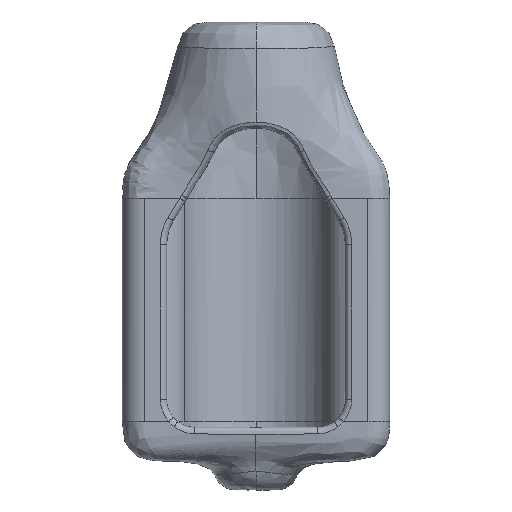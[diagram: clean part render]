
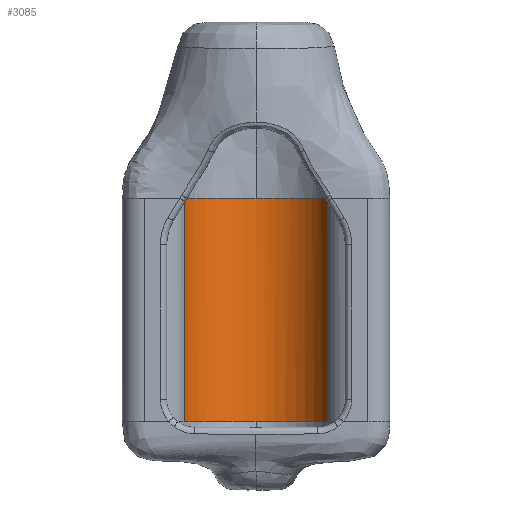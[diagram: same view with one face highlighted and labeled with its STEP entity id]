
A CAD part, front view. The second image highlights one B-rep face of the part: STEP entity #3085.
In plain terms, the highlighted cylindrical face has radius 5.334 mm (diameter 10.668 mm), a partial arc.
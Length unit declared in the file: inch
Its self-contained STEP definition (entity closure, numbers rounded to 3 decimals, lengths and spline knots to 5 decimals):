
#1007 = CARTESIAN_POINT ( 'NONE',  ( -0.13242, 0.16425, 0.3 ) ) ;
#1237 = CARTESIAN_POINT ( 'NONE',  ( -0.09839, 0.18664, 0.3 ) ) ;
#2120 = ORIENTED_EDGE ( 'NONE', *, *, #5788, .F. ) ;
#2580 = B_SPLINE_CURVE_WITH_KNOTS ( 'NONE', 3,
 ( #12126, #18629, #8421, #4940, #1237, #1007, #15390, #19093, #15161, #11673 ),
 .UNSPECIFIED., .F., .F.,
 ( 4, 2, 2, 2, 4 ),
 ( 0., 0.25, 0.5, 0.75, 1. ),
 .UNSPECIFIED. ) ;
#3085 = ADVANCED_FACE ( 'NONE', ( #8652 ), #4949, .F. ) ;
#3102 = CARTESIAN_POINT ( 'NONE',  ( -0.19284, 0.08315, 0. ) ) ;
#3158 = CARTESIAN_POINT ( 'NONE',  ( -0.17781, 0.11334, -0.3 ) ) ;
#3614 = CARTESIAN_POINT ( 'NONE',  ( -0.10339, 0.18471, -0.3 ) ) ;
#4940 = CARTESIAN_POINT ( 'NONE',  ( -0.07974, 0.19533, 0.3 ) ) ;
#4949 = CYLINDRICAL_SURFACE ( 'NONE', #31239, 0.21 ) ;
#5514 = CARTESIAN_POINT ( 'NONE',  ( 0.14779, 0.15057, 0.3 ) ) ;
#5788 = EDGE_CURVE ( 'NONE', #8398, #17415, #29320, .T. ) ;
#6465 = CARTESIAN_POINT ( 'NONE',  ( 0.19284, 0.08315, 0.3 ) ) ;
#8117 = VERTEX_POINT ( 'NONE', #12225 ) ;
#8315 = CARTESIAN_POINT ( 'NONE',  ( 0., 0.21, 0.3 ) ) ;
#8361 = EDGE_CURVE ( 'NONE', #17415, #32532, #33169, .T. ) ;
#8390 = ORIENTED_EDGE ( 'NONE', *, *, #43755, .T. ) ;
#8398 = VERTEX_POINT ( 'NONE', #17536 ) ;
#8421 = CARTESIAN_POINT ( 'NONE',  ( -0.04073, 0.20702, 0.3 ) ) ;
#8652 = FACE_OUTER_BOUND ( 'NONE', #40180, .T. ) ;
#8676 = B_SPLINE_CURVE_WITH_KNOTS ( 'NONE', 3,
 ( #37296, #40773, #43806, #5514, #16187, #44489, #39868, #43579, #36384, #8315 ),
 .UNSPECIFIED., .F., .F.,
 ( 4, 2, 2, 2, 4 ),
 ( 0., 0.25, 0.5, 0.75, 1. ),
 .UNSPECIFIED. ) ;
#8844 = ORIENTED_EDGE ( 'NONE', *, *, #27323, .T. ) ;
#9076 = CARTESIAN_POINT ( 'NONE',  ( 0.18831, 0.09364, -0.3 ) ) ;
#11673 = CARTESIAN_POINT ( 'NONE',  ( -0.19284, 0.08315, 0.3 ) ) ;
#12126 = CARTESIAN_POINT ( 'NONE',  ( 0., 0.21, 0.3 ) ) ;
#12184 = CARTESIAN_POINT ( 'NONE',  ( 0.19284, 0.08315, 0. ) ) ;
#12225 = CARTESIAN_POINT ( 'NONE',  ( -0.19284, 0.08315, 0.3 ) ) ;
#12360 = DIRECTION ( 'NONE',  ( 1., 0., 0. ) ) ;
#13601 = CARTESIAN_POINT ( 'NONE',  ( -0.18831, 0.09364, -0.3 ) ) ;
#14013 = LINE ( 'NONE', #3102, #37925 ) ;
#15161 = CARTESIAN_POINT ( 'NONE',  ( -0.18477, 0.10185, 0.3 ) ) ;
#15390 = CARTESIAN_POINT ( 'NONE',  ( -0.14779, 0.15057, 0.3 ) ) ;
#16187 = CARTESIAN_POINT ( 'NONE',  ( 0.13242, 0.16425, 0.3 ) ) ;
#16733 = CARTESIAN_POINT ( 'NONE',  ( 0.17781, 0.11334, -0.3 ) ) ;
#16959 = CARTESIAN_POINT ( 'NONE',  ( 0.01932, 0.21, -0.3 ) ) ;
#17415 = VERTEX_POINT ( 'NONE', #38245 ) ;
#17536 = CARTESIAN_POINT ( 'NONE',  ( 0.19284, 0.08315, -0.3 ) ) ;
#17591 = VERTEX_POINT ( 'NONE', #6465 ) ;
#18629 = CARTESIAN_POINT ( 'NONE',  ( -0.02036, 0.21, 0.3 ) ) ;
#18925 = CARTESIAN_POINT ( 'NONE',  ( -0.19284, 0.08315, -0.3 ) ) ;
#19093 = CARTESIAN_POINT ( 'NONE',  ( -0.17397, 0.11937, 0.3 ) ) ;
#19153 = LINE ( 'NONE', #12184, #31270 ) ;
#20446 = CARTESIAN_POINT ( 'NONE',  ( 0.05795, 0.20467, -0.3 ) ) ;
#20845 = ORIENTED_EDGE ( 'NONE', *, *, #8361, .F. ) ;
#21021 = CARTESIAN_POINT ( 'NONE',  ( -0.15842, 0.13904, -0.3 ) ) ;
#21658 = DIRECTION ( 'NONE',  ( 0., 0., 1. ) ) ;
#23000 = CARTESIAN_POINT ( 'NONE',  ( 0., 0.21, -0.3 ) ) ;
#24727 = CARTESIAN_POINT ( 'NONE',  ( -0.13617, 0.16085, -0.3 ) ) ;
#25954 = EDGE_CURVE ( 'NONE', #32532, #8117, #14013, .T. ) ;
#26335 = DIRECTION ( 'NONE',  ( 0., 0., 1. ) ) ;
#27323 = EDGE_CURVE ( 'NONE', #33385, #8117, #2580, .T. ) ;
#29320 = B_SPLINE_CURVE_WITH_KNOTS ( 'NONE', 3,
 ( #40858, #9076, #16733, #34366, #40628, #44346, #20446, #16959, #23000 ),
 .UNSPECIFIED., .F., .F.,
 ( 4, 1, 1, 1, 1, 1, 4 ),
 ( 0., 0.0625, 0.125, 0.1875, 0.25, 0.375, 0.5 ),
 .UNSPECIFIED. ) ;
#30225 = CARTESIAN_POINT ( 'NONE',  ( 0., 0., 0. ) ) ;
#30779 = CARTESIAN_POINT ( 'NONE',  ( 0., 0.21, -0.3 ) ) ;
#31231 = CARTESIAN_POINT ( 'NONE',  ( -0.19284, 0.08315, -0.3 ) ) ;
#31239 = AXIS2_PLACEMENT_3D ( 'NONE', #30225, #44373, #12360 ) ;
#31270 = VECTOR ( 'NONE', #26335, 39.37008 ) ;
#32532 = VERTEX_POINT ( 'NONE', #18925 ) ;
#33169 = B_SPLINE_CURVE_WITH_KNOTS ( 'NONE', 3,
 ( #30779, #44928, #40523, #3614, #24727, #21021, #3158, #13601, #31231 ),
 .UNSPECIFIED., .F., .F.,
 ( 4, 1, 1, 1, 1, 1, 4 ),
 ( 0.5, 0.625, 0.75, 0.8125, 0.875, 0.9375, 1. ),
 .UNSPECIFIED. ) ;
#33385 = VERTEX_POINT ( 'NONE', #40707 ) ;
#34366 = CARTESIAN_POINT ( 'NONE',  ( 0.15842, 0.13904, -0.3 ) ) ;
#35854 = EDGE_CURVE ( 'NONE', #17591, #33385, #8676, .T. ) ;
#36384 = CARTESIAN_POINT ( 'NONE',  ( 0.02036, 0.21, 0.3 ) ) ;
#37296 = CARTESIAN_POINT ( 'NONE',  ( 0.19284, 0.08315, 0.3 ) ) ;
#37368 = ORIENTED_EDGE ( 'NONE', *, *, #25954, .F. ) ;
#37925 = VECTOR ( 'NONE', #21658, 39.37008 ) ;
#38245 = CARTESIAN_POINT ( 'NONE',  ( 0., 0.21, -0.3 ) ) ;
#39868 = CARTESIAN_POINT ( 'NONE',  ( 0.07974, 0.19533, 0.3 ) ) ;
#40180 = EDGE_LOOP ( 'NONE', ( #8844, #37368, #20845, #2120, #8390, #45716 ) ) ;
#40523 = CARTESIAN_POINT ( 'NONE',  ( -0.05795, 0.20467, -0.3 ) ) ;
#40628 = CARTESIAN_POINT ( 'NONE',  ( 0.13617, 0.16085, -0.3 ) ) ;
#40707 = CARTESIAN_POINT ( 'NONE',  ( 0., 0.21, 0.3 ) ) ;
#40773 = CARTESIAN_POINT ( 'NONE',  ( 0.18477, 0.10185, 0.3 ) ) ;
#40858 = CARTESIAN_POINT ( 'NONE',  ( 0.19284, 0.08315, -0.3 ) ) ;
#43579 = CARTESIAN_POINT ( 'NONE',  ( 0.04073, 0.20702, 0.3 ) ) ;
#43755 = EDGE_CURVE ( 'NONE', #8398, #17591, #19153, .T. ) ;
#43806 = CARTESIAN_POINT ( 'NONE',  ( 0.17397, 0.11937, 0.3 ) ) ;
#44346 = CARTESIAN_POINT ( 'NONE',  ( 0.10339, 0.18471, -0.3 ) ) ;
#44373 = DIRECTION ( 'NONE',  ( 0., 0., 1. ) ) ;
#44489 = CARTESIAN_POINT ( 'NONE',  ( 0.09839, 0.18664, 0.3 ) ) ;
#44928 = CARTESIAN_POINT ( 'NONE',  ( -0.01932, 0.21, -0.3 ) ) ;
#45716 = ORIENTED_EDGE ( 'NONE', *, *, #35854, .T. ) ;
